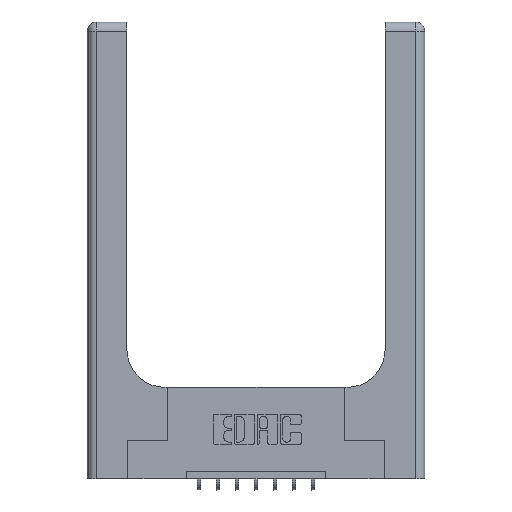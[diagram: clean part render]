
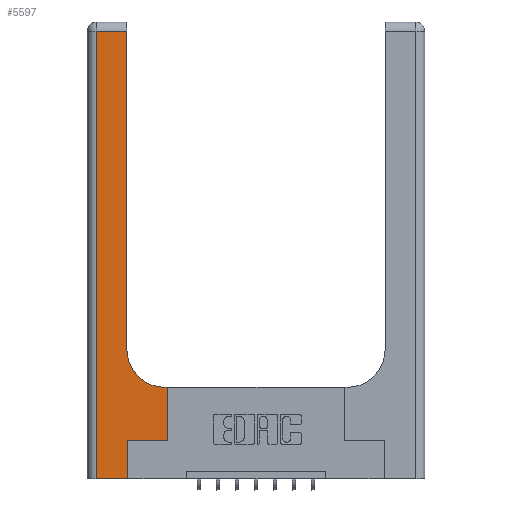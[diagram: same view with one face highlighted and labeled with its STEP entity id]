
A CAD part, top view. The second image highlights one B-rep face of the part: STEP entity #5597.
In plain terms, the highlighted planar face has unit normal (0, 0, 1).
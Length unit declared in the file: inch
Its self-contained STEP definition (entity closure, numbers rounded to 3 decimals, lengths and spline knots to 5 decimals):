
#184 = CARTESIAN_POINT ( 'NONE',  ( 0., 2.94, 0.37 ) ) ;
#449 = VERTEX_POINT ( 'NONE', #8537 ) ;
#466 = CARTESIAN_POINT ( 'NONE',  ( 0.528, 0.6, 0.37 ) ) ;
#580 = LINE ( 'NONE', #14056, #6295 ) ;
#912 = DIRECTION ( 'NONE',  ( 1., 0., 0. ) ) ;
#1178 = DIRECTION ( 'NONE',  ( 0., 0., -1. ) ) ;
#1280 = ORIENTED_EDGE ( 'NONE', *, *, #1868, .T. ) ;
#1338 = ORIENTED_EDGE ( 'NONE', *, *, #10942, .T. ) ;
#1819 = AXIS2_PLACEMENT_3D ( 'NONE', #9988, #3416, #11089 ) ;
#1827 = CARTESIAN_POINT ( 'NONE',  ( 0.265, 0., 0.37 ) ) ;
#1868 = EDGE_CURVE ( 'NONE', #14196, #8038, #11728, .T. ) ;
#1929 = ORIENTED_EDGE ( 'NONE', *, *, #9803, .T. ) ;
#2194 = CARTESIAN_POINT ( 'NONE',  ( 0.265, 0.25, 0.37 ) ) ;
#2247 = PLANE ( 'NONE',  #1819 ) ;
#2293 = DIRECTION ( 'NONE',  ( 0., -1., 0. ) ) ;
#2487 = LINE ( 'NONE', #5029, #10944 ) ;
#2659 = DIRECTION ( 'NONE',  ( 0., 1., 0. ) ) ;
#2689 = LINE ( 'NONE', #3602, #8528 ) ;
#3265 = FACE_OUTER_BOUND ( 'NONE', #9506, .T. ) ;
#3416 = DIRECTION ( 'NONE',  ( 0., 0., -1. ) ) ;
#3563 = VERTEX_POINT ( 'NONE', #1827 ) ;
#3602 = CARTESIAN_POINT ( 'NONE',  ( 0.26, 3., 0.37 ) ) ;
#3932 = DIRECTION ( 'NONE',  ( -1., 0., 0. ) ) ;
#4119 = ORIENTED_EDGE ( 'NONE', *, *, #10323, .T. ) ;
#4183 = DIRECTION ( 'NONE',  ( 0., 1., 0. ) ) ;
#4697 = VECTOR ( 'NONE', #9188, 39.37008 ) ;
#4826 = EDGE_CURVE ( 'NONE', #10241, #9168, #6395, .T. ) ;
#4968 = EDGE_CURVE ( 'NONE', #5579, #7979, #13001, .T. ) ;
#5029 = CARTESIAN_POINT ( 'NONE',  ( 0.26, 0.6, 0.37 ) ) ;
#5579 = VERTEX_POINT ( 'NONE', #2194 ) ;
#5597 = ADVANCED_FACE ( 'NONE', ( #3265 ), #2247, .F. ) ;
#6223 = CARTESIAN_POINT ( 'NONE',  ( 0.26, 0.85, 0.37 ) ) ;
#6295 = VECTOR ( 'NONE', #912, 39.37008 ) ;
#6395 = LINE ( 'NONE', #7815, #11847 ) ;
#6473 = DIRECTION ( 'NONE',  ( 1., 0., 0. ) ) ;
#6941 = VECTOR ( 'NONE', #4183, 39.37008 ) ;
#6955 = VERTEX_POINT ( 'NONE', #466 ) ;
#7194 = AXIS2_PLACEMENT_3D ( 'NONE', #7905, #1178, #8991 ) ;
#7650 = VECTOR ( 'NONE', #2659, 39.37008 ) ;
#7748 = ORIENTED_EDGE ( 'NONE', *, *, #9067, .T. ) ;
#7815 = CARTESIAN_POINT ( 'NONE',  ( 0.06, 3., 0.37 ) ) ;
#7895 = ORIENTED_EDGE ( 'NONE', *, *, #12385, .T. ) ;
#7905 = CARTESIAN_POINT ( 'NONE',  ( 0.51, 0.85, 0.37 ) ) ;
#7979 = VERTEX_POINT ( 'NONE', #13695 ) ;
#8038 = VERTEX_POINT ( 'NONE', #6223 ) ;
#8528 = VECTOR ( 'NONE', #10180, 39.37008 ) ;
#8537 = CARTESIAN_POINT ( 'NONE',  ( 0.26, 2.94, 0.37 ) ) ;
#8991 = DIRECTION ( 'NONE',  ( 1., 0., 0. ) ) ;
#9067 = EDGE_CURVE ( 'NONE', #8038, #449, #2689, .T. ) ;
#9168 = VERTEX_POINT ( 'NONE', #13760 ) ;
#9188 = DIRECTION ( 'NONE',  ( -1., 0., 0. ) ) ;
#9197 = CARTESIAN_POINT ( 'NONE',  ( 0.51, 0.6, 0.37 ) ) ;
#9506 = EDGE_LOOP ( 'NONE', ( #7748, #11758, #9594, #1338, #4119, #12341, #7895, #1929, #1280 ) ) ;
#9594 = ORIENTED_EDGE ( 'NONE', *, *, #4826, .T. ) ;
#9803 = EDGE_CURVE ( 'NONE', #6955, #14196, #2487, .T. ) ;
#9988 = CARTESIAN_POINT ( 'NONE',  ( 0., 3., 0.37 ) ) ;
#10180 = DIRECTION ( 'NONE',  ( 0., 1., 0. ) ) ;
#10241 = VERTEX_POINT ( 'NONE', #12360 ) ;
#10323 = EDGE_CURVE ( 'NONE', #3563, #5579, #10607, .T. ) ;
#10389 = CARTESIAN_POINT ( 'NONE',  ( 0.265, 0., 0.37 ) ) ;
#10607 = LINE ( 'NONE', #10389, #7650 ) ;
#10748 = CARTESIAN_POINT ( 'NONE',  ( 0.528, 0.25, 0.37 ) ) ;
#10844 = VECTOR ( 'NONE', #6473, 39.37008 ) ;
#10942 = EDGE_CURVE ( 'NONE', #9168, #3563, #580, .T. ) ;
#10944 = VECTOR ( 'NONE', #3932, 39.37008 ) ;
#11089 = DIRECTION ( 'NONE',  ( -1., 0., 0. ) ) ;
#11728 = CIRCLE ( 'NONE', #7194, 0.25 ) ;
#11758 = ORIENTED_EDGE ( 'NONE', *, *, #12794, .T. ) ;
#11847 = VECTOR ( 'NONE', #2293, 39.37008 ) ;
#11892 = CARTESIAN_POINT ( 'NONE',  ( 0.265, 0.25, 0.37 ) ) ;
#12341 = ORIENTED_EDGE ( 'NONE', *, *, #4968, .T. ) ;
#12360 = CARTESIAN_POINT ( 'NONE',  ( 0.06, 2.94, 0.37 ) ) ;
#12385 = EDGE_CURVE ( 'NONE', #7979, #6955, #12389, .T. ) ;
#12389 = LINE ( 'NONE', #10748, #6941 ) ;
#12794 = EDGE_CURVE ( 'NONE', #449, #10241, #13356, .T. ) ;
#13001 = LINE ( 'NONE', #11892, #10844 ) ;
#13356 = LINE ( 'NONE', #184, #4697 ) ;
#13695 = CARTESIAN_POINT ( 'NONE',  ( 0.528, 0.25, 0.37 ) ) ;
#13760 = CARTESIAN_POINT ( 'NONE',  ( 0.06, 0., 0.37 ) ) ;
#14056 = CARTESIAN_POINT ( 'NONE',  ( 0., 0., 0.37 ) ) ;
#14196 = VERTEX_POINT ( 'NONE', #9197 ) ;
